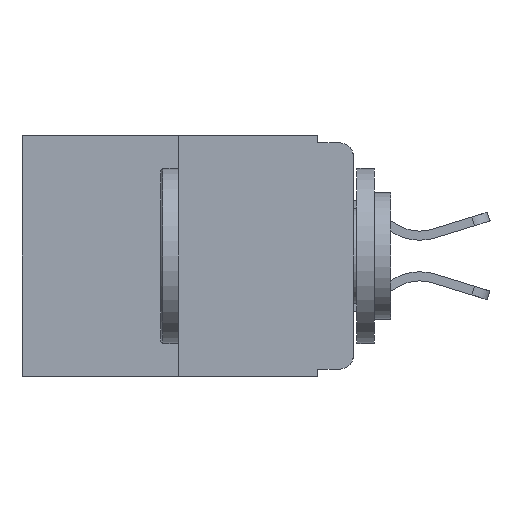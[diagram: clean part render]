
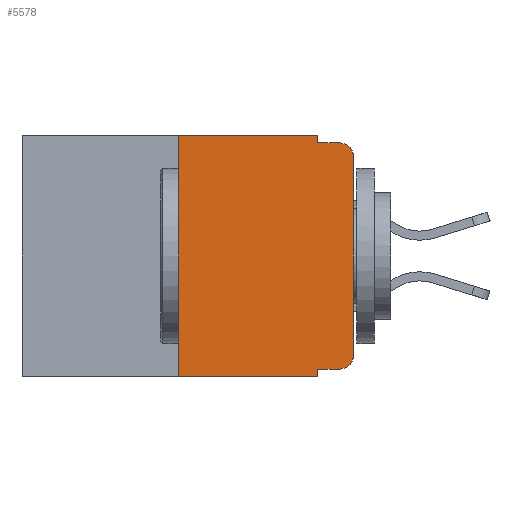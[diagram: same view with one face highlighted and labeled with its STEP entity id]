
A CAD part, left-side view. The second image highlights one B-rep face of the part: STEP entity #5578.
In plain terms, the highlighted planar face has unit normal (-1, 0, 0).
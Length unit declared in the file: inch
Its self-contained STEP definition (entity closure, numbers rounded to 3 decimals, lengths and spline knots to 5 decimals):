
#101 = DIRECTION ( 'NONE',  ( 0., 0., 1. ) ) ;
#151 = LINE ( 'NONE', #6394, #24266 ) ;
#208 = CIRCLE ( 'NONE', #6220, 0.02 ) ;
#259 = DIRECTION ( 'NONE',  ( 0., 0., -1. ) ) ;
#432 = CARTESIAN_POINT ( 'NONE',  ( 0., 0.473, -0.343 ) ) ;
#707 = DIRECTION ( 'NONE',  ( 1., 0., 0. ) ) ;
#791 = CARTESIAN_POINT ( 'NONE',  ( 0., 0.051, -0.333 ) ) ;
#806 = ORIENTED_EDGE ( 'NONE', *, *, #5443, .T. ) ;
#979 = CARTESIAN_POINT ( 'NONE',  ( 0., 0.051, 0. ) ) ;
#2358 = AXIS2_PLACEMENT_3D ( 'NONE', #8690, #707, #4624 ) ;
#2706 = EDGE_CURVE ( 'NONE', #16032, #20651, #4663, .T. ) ;
#2843 = DIRECTION ( 'NONE',  ( 0., 0., 1. ) ) ;
#2856 = CARTESIAN_POINT ( 'NONE',  ( 0., 0.02, -0.03 ) ) ;
#2876 = CARTESIAN_POINT ( 'NONE',  ( 0., 0.25, -0.343 ) ) ;
#3075 = VECTOR ( 'NONE', #5054, 39.37008 ) ;
#3649 = LINE ( 'NONE', #432, #21733 ) ;
#4624 = DIRECTION ( 'NONE',  ( 0., 0., -1. ) ) ;
#4663 = LINE ( 'NONE', #21520, #3075 ) ;
#4786 = CARTESIAN_POINT ( 'NONE',  ( 0., 0.25, 0. ) ) ;
#4939 = ORIENTED_EDGE ( 'NONE', *, *, #19601, .F. ) ;
#5054 = DIRECTION ( 'NONE',  ( 0., -1., 0. ) ) ;
#5443 = EDGE_CURVE ( 'NONE', #23016, #15097, #7097, .T. ) ;
#5578 = ADVANCED_FACE ( 'NONE', ( #9931 ), #6584, .F. ) ;
#5863 = EDGE_CURVE ( 'NONE', #21755, #23016, #8965, .T. ) ;
#6220 = AXIS2_PLACEMENT_3D ( 'NONE', #2856, #14900, #8953 ) ;
#6371 = CARTESIAN_POINT ( 'NONE',  ( 0., 0.051, -0.343 ) ) ;
#6394 = CARTESIAN_POINT ( 'NONE',  ( 0., 0.051, 0. ) ) ;
#6584 = PLANE ( 'NONE',  #2358 ) ;
#6736 = DIRECTION ( 'NONE',  ( 0., -1., 0. ) ) ;
#7097 = LINE ( 'NONE', #18403, #10558 ) ;
#7553 = VERTEX_POINT ( 'NONE', #6371 ) ;
#7663 = CARTESIAN_POINT ( 'NONE',  ( 0., 0.051, -0.01 ) ) ;
#8690 = CARTESIAN_POINT ( 'NONE',  ( 0., 0.473, 0. ) ) ;
#8691 = CARTESIAN_POINT ( 'NONE',  ( 0., 0.051, 0. ) ) ;
#8953 = DIRECTION ( 'NONE',  ( 0., 0., -1. ) ) ;
#8965 = CIRCLE ( 'NONE', #21376, 0.02 ) ;
#9266 = VERTEX_POINT ( 'NONE', #791 ) ;
#9771 = EDGE_CURVE ( 'NONE', #9266, #7553, #26111, .T. ) ;
#9791 = VERTEX_POINT ( 'NONE', #2876 ) ;
#9931 = FACE_OUTER_BOUND ( 'NONE', #22790, .T. ) ;
#9959 = DIRECTION ( 'NONE',  ( -1., 0., 0. ) ) ;
#10558 = VECTOR ( 'NONE', #101, 39.37008 ) ;
#10635 = EDGE_CURVE ( 'NONE', #9266, #21755, #23511, .T. ) ;
#11076 = VECTOR ( 'NONE', #14091, 39.37008 ) ;
#11122 = VERTEX_POINT ( 'NONE', #11743 ) ;
#11743 = CARTESIAN_POINT ( 'NONE',  ( 0., 0.02, -0.01 ) ) ;
#12347 = ORIENTED_EDGE ( 'NONE', *, *, #2706, .F. ) ;
#12366 = LINE ( 'NONE', #15872, #11076 ) ;
#12810 = DIRECTION ( 'NONE',  ( 0., 0., -1. ) ) ;
#13094 = ORIENTED_EDGE ( 'NONE', *, *, #9771, .F. ) ;
#13693 = CARTESIAN_POINT ( 'NONE',  ( 0., 0.02, -0.313 ) ) ;
#14091 = DIRECTION ( 'NONE',  ( 0., -1., 0. ) ) ;
#14236 = CARTESIAN_POINT ( 'NONE',  ( 0., 0.02, -0.333 ) ) ;
#14900 = DIRECTION ( 'NONE',  ( -1., 0., 0. ) ) ;
#15097 = VERTEX_POINT ( 'NONE', #21178 ) ;
#15360 = LINE ( 'NONE', #4786, #25829 ) ;
#15381 = ORIENTED_EDGE ( 'NONE', *, *, #22846, .F. ) ;
#15872 = CARTESIAN_POINT ( 'NONE',  ( 0., 0.051, -0.01 ) ) ;
#16032 = VERTEX_POINT ( 'NONE', #17979 ) ;
#17050 = EDGE_CURVE ( 'NONE', #9791, #7553, #3649, .T. ) ;
#17785 = ORIENTED_EDGE ( 'NONE', *, *, #24447, .T. ) ;
#17952 = VERTEX_POINT ( 'NONE', #7663 ) ;
#17979 = CARTESIAN_POINT ( 'NONE',  ( 0., 0.25, 0. ) ) ;
#18005 = ORIENTED_EDGE ( 'NONE', *, *, #18741, .F. ) ;
#18403 = CARTESIAN_POINT ( 'NONE',  ( 0., 0., 0. ) ) ;
#18621 = CARTESIAN_POINT ( 'NONE',  ( 0., 0., -0.313 ) ) ;
#18741 = EDGE_CURVE ( 'NONE', #20651, #17952, #151, .T. ) ;
#19124 = VECTOR ( 'NONE', #24761, 39.37008 ) ;
#19416 = ORIENTED_EDGE ( 'NONE', *, *, #10635, .T. ) ;
#19601 = EDGE_CURVE ( 'NONE', #9791, #16032, #15360, .T. ) ;
#20076 = DIRECTION ( 'NONE',  ( 0., 0., -1. ) ) ;
#20651 = VERTEX_POINT ( 'NONE', #8691 ) ;
#21178 = CARTESIAN_POINT ( 'NONE',  ( 0., 0., -0.03 ) ) ;
#21376 = AXIS2_PLACEMENT_3D ( 'NONE', #13693, #9959, #20076 ) ;
#21520 = CARTESIAN_POINT ( 'NONE',  ( 0., 0.473, 0. ) ) ;
#21521 = ORIENTED_EDGE ( 'NONE', *, *, #17050, .T. ) ;
#21733 = VECTOR ( 'NONE', #6736, 39.37008 ) ;
#21755 = VERTEX_POINT ( 'NONE', #14236 ) ;
#22790 = EDGE_LOOP ( 'NONE', ( #806, #17785, #15381, #18005, #12347, #4939, #21521, #13094, #19416, #23509 ) ) ;
#22846 = EDGE_CURVE ( 'NONE', #17952, #11122, #12366, .T. ) ;
#23016 = VERTEX_POINT ( 'NONE', #18621 ) ;
#23509 = ORIENTED_EDGE ( 'NONE', *, *, #5863, .T. ) ;
#23511 = LINE ( 'NONE', #26022, #19124 ) ;
#23869 = VECTOR ( 'NONE', #12810, 39.37008 ) ;
#24266 = VECTOR ( 'NONE', #259, 39.37008 ) ;
#24447 = EDGE_CURVE ( 'NONE', #15097, #11122, #208, .T. ) ;
#24761 = DIRECTION ( 'NONE',  ( 0., -1., 0. ) ) ;
#25829 = VECTOR ( 'NONE', #2843, 39.37008 ) ;
#26022 = CARTESIAN_POINT ( 'NONE',  ( 0., 0.051, -0.333 ) ) ;
#26111 = LINE ( 'NONE', #979, #23869 ) ;
